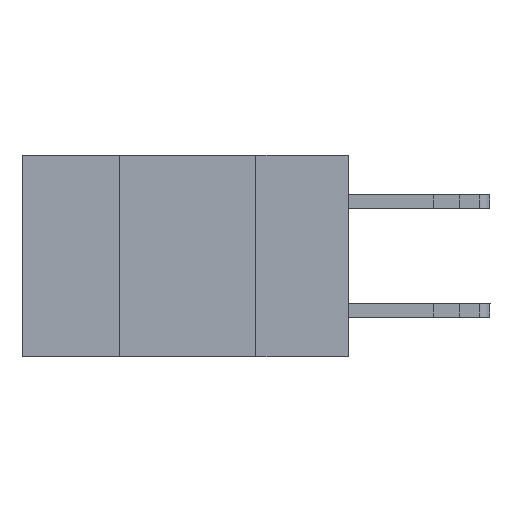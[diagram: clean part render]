
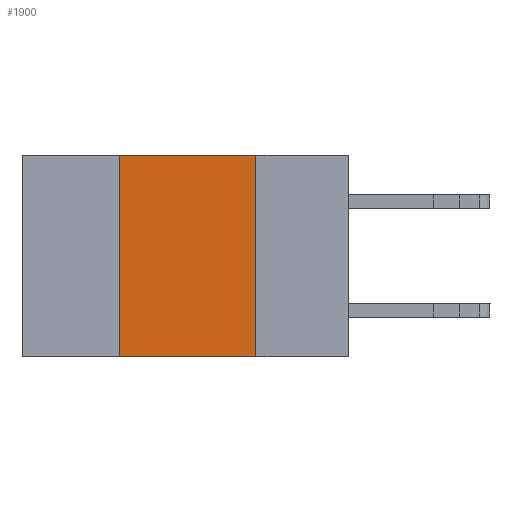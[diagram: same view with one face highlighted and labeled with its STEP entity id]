
A CAD part, left-side view. The second image highlights one B-rep face of the part: STEP entity #1900.
In plain terms, the highlighted planar face has unit normal (-1, 0, 0).
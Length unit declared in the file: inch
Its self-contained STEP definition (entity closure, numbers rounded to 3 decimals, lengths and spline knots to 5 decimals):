
#202 = ORIENTED_EDGE ( 'NONE', *, *, #13912, .T. ) ;
#394 = EDGE_CURVE ( 'NONE', #8844, #475, #1022, .T. ) ;
#475 = VERTEX_POINT ( 'NONE', #8268 ) ;
#602 = CARTESIAN_POINT ( 'NONE',  ( 0., 0.6, -0.37 ) ) ;
#860 = DIRECTION ( 'NONE',  ( 0., 0., -1. ) ) ;
#1022 = LINE ( 'NONE', #3296, #1396 ) ;
#1028 = DIRECTION ( 'NONE',  ( 1., 0., 0. ) ) ;
#1281 = PLANE ( 'NONE',  #6976 ) ;
#1396 = VECTOR ( 'NONE', #8395, 39.37008 ) ;
#1512 = CARTESIAN_POINT ( 'NONE',  ( 0., 0.6, 0. ) ) ;
#1801 = DIRECTION ( 'NONE',  ( 0., -1., 0. ) ) ;
#1900 = ADVANCED_FACE ( 'NONE', ( #10699 ), #1281, .F. ) ;
#2364 = CARTESIAN_POINT ( 'NONE',  ( 0., 0.42, -0.37 ) ) ;
#3041 = VECTOR ( 'NONE', #11620, 39.37008 ) ;
#3196 = EDGE_CURVE ( 'NONE', #475, #8309, #9915, .T. ) ;
#3296 = CARTESIAN_POINT ( 'NONE',  ( 0., 0.6, 0. ) ) ;
#5894 = CARTESIAN_POINT ( 'NONE',  ( 0., 0.17, -0.37 ) ) ;
#6236 = LINE ( 'NONE', #9513, #9512 ) ;
#6976 = AXIS2_PLACEMENT_3D ( 'NONE', #1512, #1028, #860 ) ;
#7123 = VERTEX_POINT ( 'NONE', #2364 ) ;
#7867 = ORIENTED_EDGE ( 'NONE', *, *, #3196, .F. ) ;
#8268 = CARTESIAN_POINT ( 'NONE',  ( 0., 0.17, 0. ) ) ;
#8309 = VERTEX_POINT ( 'NONE', #5894 ) ;
#8395 = DIRECTION ( 'NONE',  ( 0., -1., 0. ) ) ;
#8701 = EDGE_LOOP ( 'NONE', ( #7867, #11127, #14503, #202 ) ) ;
#8844 = VERTEX_POINT ( 'NONE', #12042 ) ;
#9512 = VECTOR ( 'NONE', #15196, 39.37008 ) ;
#9513 = CARTESIAN_POINT ( 'NONE',  ( 0., 0.42, -0.37 ) ) ;
#9915 = LINE ( 'NONE', #10950, #3041 ) ;
#10699 = FACE_OUTER_BOUND ( 'NONE', #8701, .T. ) ;
#10950 = CARTESIAN_POINT ( 'NONE',  ( 0., 0.17, -0.37 ) ) ;
#11127 = ORIENTED_EDGE ( 'NONE', *, *, #394, .F. ) ;
#11620 = DIRECTION ( 'NONE',  ( 0., 0., -1. ) ) ;
#12042 = CARTESIAN_POINT ( 'NONE',  ( 0., 0.42, 0. ) ) ;
#12213 = VECTOR ( 'NONE', #1801, 39.37008 ) ;
#13912 = EDGE_CURVE ( 'NONE', #7123, #8309, #15153, .T. ) ;
#14503 = ORIENTED_EDGE ( 'NONE', *, *, #14634, .F. ) ;
#14634 = EDGE_CURVE ( 'NONE', #7123, #8844, #6236, .T. ) ;
#15153 = LINE ( 'NONE', #602, #12213 ) ;
#15196 = DIRECTION ( 'NONE',  ( 0., 0., 1. ) ) ;
